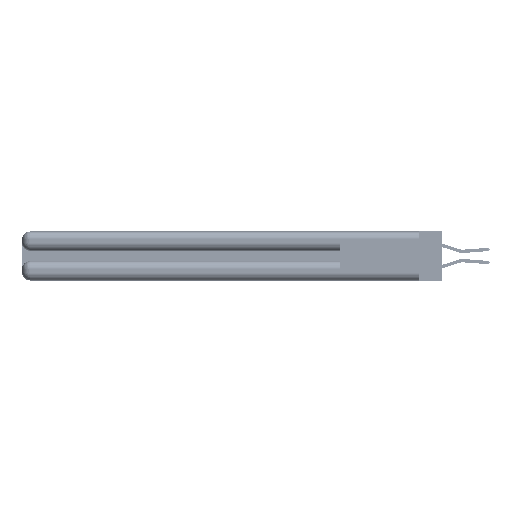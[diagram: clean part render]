
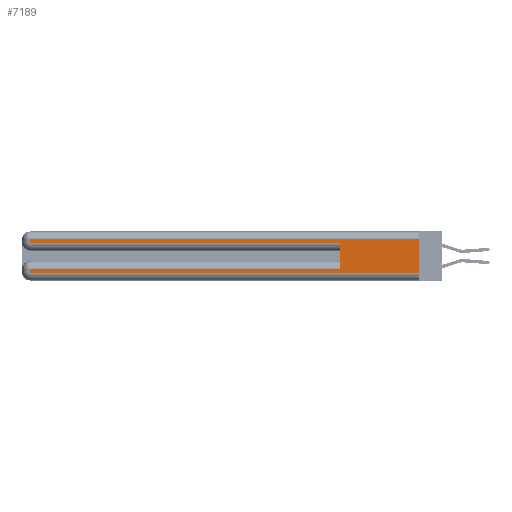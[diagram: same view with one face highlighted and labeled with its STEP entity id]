
A CAD part, left-side view. The second image highlights one B-rep face of the part: STEP entity #7189.
In plain terms, the highlighted planar face has unit normal (-1, 0, 0).
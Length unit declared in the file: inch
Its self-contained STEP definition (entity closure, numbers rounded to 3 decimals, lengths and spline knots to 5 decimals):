
#123 = CARTESIAN_POINT ( 'NONE',  ( 0., 0.6, 0.145 ) ) ;
#3135 = ORIENTED_EDGE ( 'NONE', *, *, #9352, .T. ) ;
#4753 = VERTEX_POINT ( 'NONE', #17111 ) ;
#5345 = DIRECTION ( 'NONE',  ( 1., 0., 0. ) ) ;
#5611 = VECTOR ( 'NONE', #36866, 39.37008 ) ;
#6066 = CARTESIAN_POINT ( 'NONE',  ( 0., 0., 0.37 ) ) ;
#6559 = CARTESIAN_POINT ( 'NONE',  ( 0., 2.94, 0.085 ) ) ;
#7189 = ADVANCED_FACE ( 'NONE', ( #37892 ), #18476, .F. ) ;
#8050 = VECTOR ( 'NONE', #47496, 39.37008 ) ;
#8189 = VERTEX_POINT ( 'NONE', #12039 ) ;
#9352 = EDGE_CURVE ( 'NONE', #27572, #33207, #54902, .T. ) ;
#9911 = VECTOR ( 'NONE', #39914, 39.37008 ) ;
#10218 = VECTOR ( 'NONE', #19128, 39.37008 ) ;
#11412 = EDGE_CURVE ( 'NONE', #42959, #4753, #46729, .T. ) ;
#12039 = CARTESIAN_POINT ( 'NONE',  ( 0., 0., 0.06 ) ) ;
#12295 = CARTESIAN_POINT ( 'NONE',  ( 0., 2.94, 0.37 ) ) ;
#15111 = EDGE_CURVE ( 'NONE', #42959, #8189, #29029, .T. ) ;
#15766 = VERTEX_POINT ( 'NONE', #45290 ) ;
#16067 = EDGE_CURVE ( 'NONE', #44146, #27572, #51805, .T. ) ;
#17111 = CARTESIAN_POINT ( 'NONE',  ( 0., 2.94, 0.31 ) ) ;
#17761 = LINE ( 'NONE', #48486, #50167 ) ;
#17789 = CARTESIAN_POINT ( 'NONE',  ( 0., 2.94, 0.37 ) ) ;
#18476 = PLANE ( 'NONE',  #38943 ) ;
#19128 = DIRECTION ( 'NONE',  ( 0., 1., 0. ) ) ;
#20043 = CARTESIAN_POINT ( 'NONE',  ( 0., 0.6, 0.085 ) ) ;
#21123 = ORIENTED_EDGE ( 'NONE', *, *, #16067, .T. ) ;
#21640 = LINE ( 'NONE', #123, #9911 ) ;
#21869 = CARTESIAN_POINT ( 'NONE',  ( 0., 2.94, 0.285 ) ) ;
#22215 = DIRECTION ( 'NONE',  ( 0., 0., -1. ) ) ;
#25306 = EDGE_CURVE ( 'NONE', #4753, #43078, #54702, .T. ) ;
#26297 = EDGE_CURVE ( 'NONE', #33207, #8189, #49879, .T. ) ;
#27572 = VERTEX_POINT ( 'NONE', #6559 ) ;
#28643 = CARTESIAN_POINT ( 'NONE',  ( 0., 0., 0.06 ) ) ;
#29029 = LINE ( 'NONE', #6066, #5611 ) ;
#30922 = DIRECTION ( 'NONE',  ( 0., -1., 0. ) ) ;
#32609 = VECTOR ( 'NONE', #22215, 39.37008 ) ;
#33034 = DIRECTION ( 'NONE',  ( 0., -1., 0. ) ) ;
#33207 = VERTEX_POINT ( 'NONE', #39774 ) ;
#33887 = DIRECTION ( 'NONE',  ( 0., 1., 0. ) ) ;
#34057 = ORIENTED_EDGE ( 'NONE', *, *, #15111, .F. ) ;
#36135 = DIRECTION ( 'NONE',  ( 0., 0., -1. ) ) ;
#36866 = DIRECTION ( 'NONE',  ( 0., 0., -1. ) ) ;
#37892 = FACE_OUTER_BOUND ( 'NONE', #50397, .T. ) ;
#38943 = AXIS2_PLACEMENT_3D ( 'NONE', #40371, #5345, #36135 ) ;
#38964 = ORIENTED_EDGE ( 'NONE', *, *, #53323, .F. ) ;
#39774 = CARTESIAN_POINT ( 'NONE',  ( 0., 2.94, 0.06 ) ) ;
#39914 = DIRECTION ( 'NONE',  ( 0., 0., 1. ) ) ;
#40007 = VECTOR ( 'NONE', #33887, 39.37008 ) ;
#40371 = CARTESIAN_POINT ( 'NONE',  ( 0., 0., 0.37 ) ) ;
#41025 = CARTESIAN_POINT ( 'NONE',  ( 0., 0., 0.31 ) ) ;
#42319 = ORIENTED_EDGE ( 'NONE', *, *, #51167, .T. ) ;
#42473 = ORIENTED_EDGE ( 'NONE', *, *, #26297, .T. ) ;
#42832 = CARTESIAN_POINT ( 'NONE',  ( 0., 0., 0.31 ) ) ;
#42959 = VERTEX_POINT ( 'NONE', #42832 ) ;
#43078 = VERTEX_POINT ( 'NONE', #21869 ) ;
#44146 = VERTEX_POINT ( 'NONE', #20043 ) ;
#44396 = ORIENTED_EDGE ( 'NONE', *, *, #11412, .T. ) ;
#45290 = CARTESIAN_POINT ( 'NONE',  ( 0., 0.6, 0.285 ) ) ;
#46466 = ORIENTED_EDGE ( 'NONE', *, *, #25306, .T. ) ;
#46729 = LINE ( 'NONE', #41025, #10218 ) ;
#47496 = DIRECTION ( 'NONE',  ( 0., 0., -1. ) ) ;
#48459 = VECTOR ( 'NONE', #33034, 39.37008 ) ;
#48486 = CARTESIAN_POINT ( 'NONE',  ( 0., 0., 0.285 ) ) ;
#49879 = LINE ( 'NONE', #28643, #48459 ) ;
#50167 = VECTOR ( 'NONE', #30922, 39.37008 ) ;
#50397 = EDGE_LOOP ( 'NONE', ( #34057, #44396, #46466, #42319, #38964, #21123, #3135, #42473 ) ) ;
#51167 = EDGE_CURVE ( 'NONE', #43078, #15766, #17761, .T. ) ;
#51485 = CARTESIAN_POINT ( 'NONE',  ( 0., 0., 0.085 ) ) ;
#51805 = LINE ( 'NONE', #51485, #40007 ) ;
#53323 = EDGE_CURVE ( 'NONE', #44146, #15766, #21640, .T. ) ;
#54702 = LINE ( 'NONE', #17789, #32609 ) ;
#54902 = LINE ( 'NONE', #12295, #8050 ) ;
